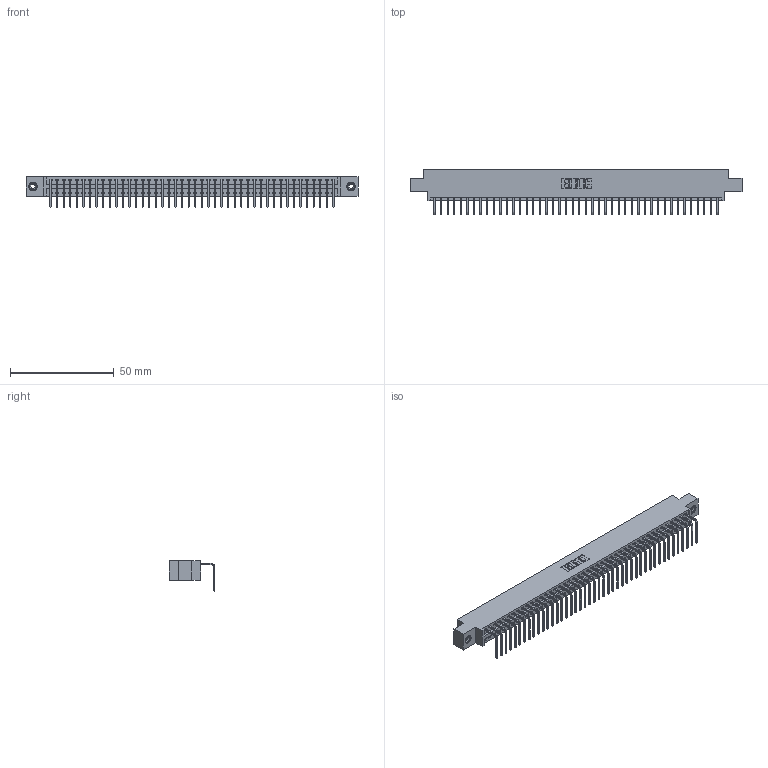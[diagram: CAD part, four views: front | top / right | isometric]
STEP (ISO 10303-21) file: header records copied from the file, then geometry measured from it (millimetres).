
FILE_DESCRIPTION (( 'STEP AP203' ), '1' );
FILE_NAME ('396-044-558-608.STEP', '2018-09-07T05:12:57', ( '' ), ( '' ), 'SwSTEP 2.0', 'SolidWorks 2016', '' );
FILE_SCHEMA (( 'CONFIG_CONTROL_DESIGN' ));
Length unit declared in the file: inch
Products named in the file (4): 346 Part_0.170 Offset - 0.156 Dia-TI; 345-292-001_558 Tail - 2; 345-250-001_345-250-003-102; 396-044-558-608
Assembly tree (47 placements, depth 2):
  396-044-558-608
    346 Part_0.170 Offset - 0.156 Dia-TI
    345-292-001_558 Tail - 2  x44
    345-250-001_345-250-003-102  x2
Bounding box: 160.27 x 22.16 x 14.73 mm (x, y, z)
Volume: 15341 mm3; surface area: 20252.6 mm2
Topology: 47 solids, 47 shells, 2826 faces, 8485 edges, 5590 vertices
Faces by surface type: plane 1960, cylinder 850, cone 12, torus 4
Entity records: 28440 total; most frequent: CARTESIAN_POINT 4859, ORIENTED_EDGE 4830, DIRECTION 4309, EDGE_CURVE 2415, LINE 2087, VECTOR 2087, VERTEX_POINT 1604, AXIS2_PLACEMENT_3D 1111
